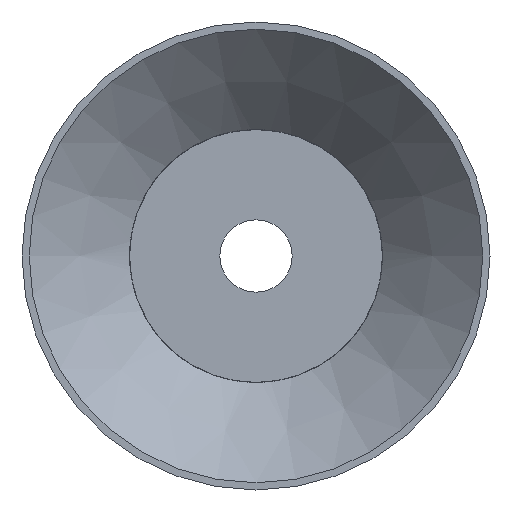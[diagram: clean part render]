
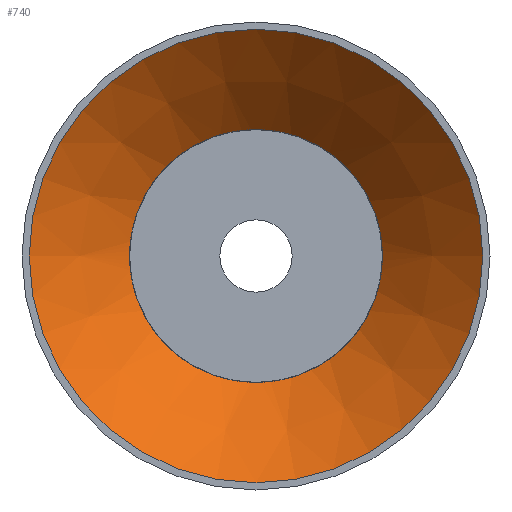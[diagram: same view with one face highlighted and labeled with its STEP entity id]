
A CAD part, front view. The second image highlights one B-rep face of the part: STEP entity #740.
In plain terms, the highlighted conical face has half-angle 44.795 degrees and reference radius 31.052 mm.
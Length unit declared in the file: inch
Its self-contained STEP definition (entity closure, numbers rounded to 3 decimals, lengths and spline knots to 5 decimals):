
#123=FACE_OUTER_BOUND('',#159,.T.);
#159=EDGE_LOOP('',(#486,#487,#488,#489,#490,#491,#492,#493,#494,#495,#496,
#497,#498));
#198=LINE('',#988,#220);
#220=VECTOR('',#852,1.2225);
#242=CIRCLE('',#791,1.57);
#243=CIRCLE('',#792,0.875);
#244=CIRCLE('',#793,0.875);
#245=CIRCLE('',#794,0.875);
#246=CIRCLE('',#795,0.875);
#247=CIRCLE('',#796,0.875);
#248=CIRCLE('',#797,0.875);
#249=CIRCLE('',#798,0.875);
#250=CIRCLE('',#799,0.875);
#251=CIRCLE('',#800,0.875);
#252=CIRCLE('',#801,1.57);
#275=VERTEX_POINT('',#984);
#276=VERTEX_POINT('',#985);
#277=VERTEX_POINT('',#987);
#278=VERTEX_POINT('',#989);
#279=VERTEX_POINT('',#991);
#280=VERTEX_POINT('',#993);
#281=VERTEX_POINT('',#995);
#282=VERTEX_POINT('',#997);
#283=VERTEX_POINT('',#999);
#284=VERTEX_POINT('',#1001);
#285=VERTEX_POINT('',#1003);
#360=EDGE_CURVE('',#275,#276,#242,.T.);
#361=EDGE_CURVE('',#276,#277,#198,.T.);
#362=EDGE_CURVE('',#278,#277,#243,.T.);
#363=EDGE_CURVE('',#279,#278,#244,.T.);
#364=EDGE_CURVE('',#280,#279,#245,.T.);
#365=EDGE_CURVE('',#281,#280,#246,.T.);
#366=EDGE_CURVE('',#282,#281,#247,.T.);
#367=EDGE_CURVE('',#283,#282,#248,.T.);
#368=EDGE_CURVE('',#284,#283,#249,.T.);
#369=EDGE_CURVE('',#285,#284,#250,.T.);
#370=EDGE_CURVE('',#277,#285,#251,.T.);
#371=EDGE_CURVE('',#276,#275,#252,.T.);
#486=ORIENTED_EDGE('',*,*,#360,.T.);
#487=ORIENTED_EDGE('',*,*,#361,.T.);
#488=ORIENTED_EDGE('',*,*,#362,.F.);
#489=ORIENTED_EDGE('',*,*,#363,.F.);
#490=ORIENTED_EDGE('',*,*,#364,.F.);
#491=ORIENTED_EDGE('',*,*,#365,.F.);
#492=ORIENTED_EDGE('',*,*,#366,.F.);
#493=ORIENTED_EDGE('',*,*,#367,.F.);
#494=ORIENTED_EDGE('',*,*,#368,.F.);
#495=ORIENTED_EDGE('',*,*,#369,.F.);
#496=ORIENTED_EDGE('',*,*,#370,.F.);
#497=ORIENTED_EDGE('',*,*,#361,.F.);
#498=ORIENTED_EDGE('',*,*,#371,.T.);
#738=CONICAL_SURFACE('',#790,1.2225,0.782);
#740=ADVANCED_FACE('',(#123),#738,.F.);
#790=AXIS2_PLACEMENT_3D('',#983,#848,#849);
#791=AXIS2_PLACEMENT_3D('',#986,#850,#851);
#792=AXIS2_PLACEMENT_3D('',#990,#853,#854);
#793=AXIS2_PLACEMENT_3D('',#992,#855,#856);
#794=AXIS2_PLACEMENT_3D('',#994,#857,#858);
#795=AXIS2_PLACEMENT_3D('',#996,#859,#860);
#796=AXIS2_PLACEMENT_3D('',#998,#861,#862);
#797=AXIS2_PLACEMENT_3D('',#1000,#863,#864);
#798=AXIS2_PLACEMENT_3D('',#1002,#865,#866);
#799=AXIS2_PLACEMENT_3D('',#1004,#867,#868);
#800=AXIS2_PLACEMENT_3D('',#1005,#869,#870);
#801=AXIS2_PLACEMENT_3D('',#1006,#871,#872);
#848=DIRECTION('center_axis',(0.,-1.,0.));
#849=DIRECTION('ref_axis',(1.,0.,0.));
#850=DIRECTION('center_axis',(0.,-1.,0.));
#851=DIRECTION('ref_axis',(1.,0.,0.));
#852=DIRECTION('',(0.705,0.71,0.));
#853=DIRECTION('center_axis',(0.,-1.,0.));
#854=DIRECTION('ref_axis',(1.,0.,0.));
#855=DIRECTION('center_axis',(0.,-1.,0.));
#856=DIRECTION('ref_axis',(1.,0.,0.));
#857=DIRECTION('center_axis',(0.,-1.,0.));
#858=DIRECTION('ref_axis',(1.,0.,0.));
#859=DIRECTION('center_axis',(0.,-1.,0.));
#860=DIRECTION('ref_axis',(1.,0.,0.));
#861=DIRECTION('center_axis',(0.,-1.,0.));
#862=DIRECTION('ref_axis',(1.,0.,0.));
#863=DIRECTION('center_axis',(0.,-1.,0.));
#864=DIRECTION('ref_axis',(1.,0.,0.));
#865=DIRECTION('center_axis',(0.,-1.,0.));
#866=DIRECTION('ref_axis',(1.,0.,0.));
#867=DIRECTION('center_axis',(0.,-1.,0.));
#868=DIRECTION('ref_axis',(1.,0.,0.));
#869=DIRECTION('center_axis',(0.,-1.,0.));
#870=DIRECTION('ref_axis',(1.,0.,0.));
#871=DIRECTION('center_axis',(0.,-1.,0.));
#872=DIRECTION('ref_axis',(1.,0.,0.));
#983=CARTESIAN_POINT('Origin',(0.,0.35,0.));
#984=CARTESIAN_POINT('',(1.57,0.,0.));
#985=CARTESIAN_POINT('',(-1.57,0.,0.));
#986=CARTESIAN_POINT('Origin',(0.,0.,0.));
#987=CARTESIAN_POINT('',(-0.875,0.7,0.));
#988=CARTESIAN_POINT('',(-1.2225,0.35,0.));
#989=CARTESIAN_POINT('',(-0.86927,0.7,0.1));
#990=CARTESIAN_POINT('Origin',(0.,0.7,0.));
#991=CARTESIAN_POINT('',(-0.1,0.7,0.86927));
#992=CARTESIAN_POINT('Origin',(0.,0.7,0.));
#993=CARTESIAN_POINT('',(0.1,0.7,0.86927));
#994=CARTESIAN_POINT('Origin',(0.,0.7,0.));
#995=CARTESIAN_POINT('',(0.86927,0.7,0.1));
#996=CARTESIAN_POINT('Origin',(0.,0.7,0.));
#997=CARTESIAN_POINT('',(0.86927,0.7,-0.1));
#998=CARTESIAN_POINT('Origin',(0.,0.7,0.));
#999=CARTESIAN_POINT('',(0.1,0.7,-0.86927));
#1000=CARTESIAN_POINT('Origin',(0.,0.7,0.));
#1001=CARTESIAN_POINT('',(-0.1,0.7,-0.86927));
#1002=CARTESIAN_POINT('Origin',(0.,0.7,0.));
#1003=CARTESIAN_POINT('',(-0.86927,0.7,-0.1));
#1004=CARTESIAN_POINT('Origin',(0.,0.7,0.));
#1005=CARTESIAN_POINT('Origin',(0.,0.7,0.));
#1006=CARTESIAN_POINT('Origin',(0.,0.,0.));
